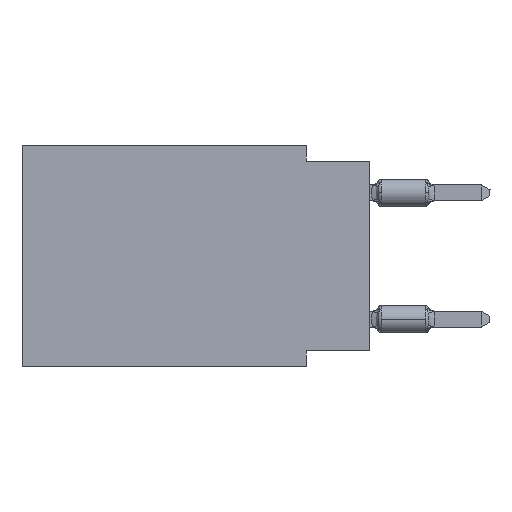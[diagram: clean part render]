
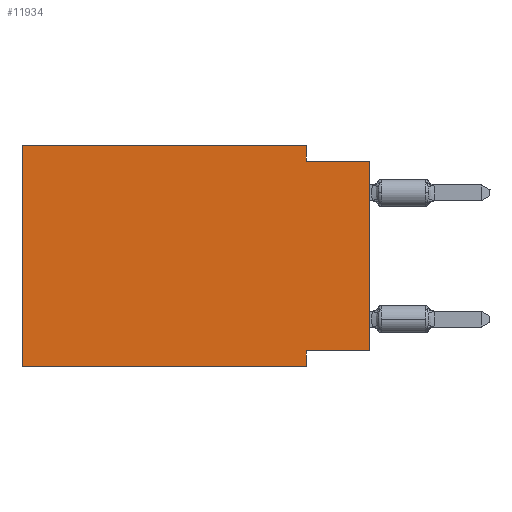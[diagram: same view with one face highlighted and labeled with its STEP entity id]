
A CAD part, left-side view. The second image highlights one B-rep face of the part: STEP entity #11934.
In plain terms, the highlighted planar face has unit normal (-1, 0, 0).
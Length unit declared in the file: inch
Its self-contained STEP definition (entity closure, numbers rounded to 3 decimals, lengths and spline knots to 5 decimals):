
#329 = CARTESIAN_POINT ( 'NONE',  ( 0., 0.55, 0. ) ) ;
#379 = DIRECTION ( 'NONE',  ( 0., -1., 0. ) ) ;
#888 = PLANE ( 'NONE',  #16378 ) ;
#1260 = DIRECTION ( 'NONE',  ( 0., 0., 1. ) ) ;
#1665 = DIRECTION ( 'NONE',  ( 0., 0., -1. ) ) ;
#2385 = EDGE_CURVE ( 'NONE', #27962, #37296, #24498, .T. ) ;
#2590 = CARTESIAN_POINT ( 'NONE',  ( 0., 0.1, 0. ) ) ;
#2630 = CARTESIAN_POINT ( 'NONE',  ( 0., 0.1, 0. ) ) ;
#3808 = CARTESIAN_POINT ( 'NONE',  ( 0., 0.1, -0.35 ) ) ;
#3850 = VERTEX_POINT ( 'NONE', #15170 ) ;
#4298 = EDGE_CURVE ( 'NONE', #32614, #6247, #18585, .T. ) ;
#4773 = EDGE_LOOP ( 'NONE', ( #17050, #33288, #7568, #12447, #37825, #22223, #14088, #26135 ) ) ;
#6037 = VERTEX_POINT ( 'NONE', #27906 ) ;
#6247 = VERTEX_POINT ( 'NONE', #2590 ) ;
#6806 = DIRECTION ( 'NONE',  ( 0., -1., 0. ) ) ;
#6886 = DIRECTION ( 'NONE',  ( 0., 0., -1. ) ) ;
#7568 = ORIENTED_EDGE ( 'NONE', *, *, #37549, .F. ) ;
#7593 = DIRECTION ( 'NONE',  ( 0., 0., 1. ) ) ;
#8701 = LINE ( 'NONE', #35371, #34907 ) ;
#9130 = VECTOR ( 'NONE', #1665, 39.37008 ) ;
#11760 = VECTOR ( 'NONE', #7593, 39.37008 ) ;
#11934 = ADVANCED_FACE ( 'NONE', ( #29723 ), #888, .F. ) ;
#12447 = ORIENTED_EDGE ( 'NONE', *, *, #4298, .F. ) ;
#12802 = LINE ( 'NONE', #31176, #11760 ) ;
#12887 = DIRECTION ( 'NONE',  ( 0., -1., 0. ) ) ;
#14088 = ORIENTED_EDGE ( 'NONE', *, *, #2385, .F. ) ;
#14455 = VECTOR ( 'NONE', #1260, 39.37008 ) ;
#14785 = DIRECTION ( 'NONE',  ( 0., 0., -1. ) ) ;
#14844 = EDGE_CURVE ( 'NONE', #34185, #6037, #36817, .T. ) ;
#15170 = CARTESIAN_POINT ( 'NONE',  ( 0., 0.55, -0.35 ) ) ;
#15378 = DIRECTION ( 'NONE',  ( 1., 0., 0. ) ) ;
#16009 = VECTOR ( 'NONE', #30143, 39.37008 ) ;
#16378 = AXIS2_PLACEMENT_3D ( 'NONE', #329, #15378, #6886 ) ;
#17050 = ORIENTED_EDGE ( 'NONE', *, *, #14844, .T. ) ;
#18198 = CARTESIAN_POINT ( 'NONE',  ( 0., 0.55, 0. ) ) ;
#18585 = LINE ( 'NONE', #19320, #33521 ) ;
#18828 = CARTESIAN_POINT ( 'NONE',  ( 0., 0., 0. ) ) ;
#18860 = CARTESIAN_POINT ( 'NONE',  ( 0., 0.1, -0.35 ) ) ;
#19320 = CARTESIAN_POINT ( 'NONE',  ( 0., 0.55, 0. ) ) ;
#19753 = VECTOR ( 'NONE', #12887, 39.37008 ) ;
#19754 = CARTESIAN_POINT ( 'NONE',  ( 0., 0., -0.325 ) ) ;
#20497 = CARTESIAN_POINT ( 'NONE',  ( 0., 0.1, -0.025 ) ) ;
#22223 = ORIENTED_EDGE ( 'NONE', *, *, #24764, .T. ) ;
#23351 = CARTESIAN_POINT ( 'NONE',  ( 0., 0.1, -0.325 ) ) ;
#24498 = LINE ( 'NONE', #18860, #9130 ) ;
#24672 = EDGE_CURVE ( 'NONE', #34185, #27962, #35767, .T. ) ;
#24764 = EDGE_CURVE ( 'NONE', #3850, #37296, #34374, .T. ) ;
#25333 = VECTOR ( 'NONE', #14785, 39.37008 ) ;
#25657 = EDGE_CURVE ( 'NONE', #3850, #32614, #12802, .T. ) ;
#26135 = ORIENTED_EDGE ( 'NONE', *, *, #24672, .F. ) ;
#26202 = LINE ( 'NONE', #2630, #25333 ) ;
#27906 = CARTESIAN_POINT ( 'NONE',  ( 0., 0., -0.025 ) ) ;
#27962 = VERTEX_POINT ( 'NONE', #23351 ) ;
#29723 = FACE_OUTER_BOUND ( 'NONE', #4773, .T. ) ;
#30143 = DIRECTION ( 'NONE',  ( 0., 1., 0. ) ) ;
#31074 = CARTESIAN_POINT ( 'NONE',  ( 0., 0.55, -0.35 ) ) ;
#31176 = CARTESIAN_POINT ( 'NONE',  ( 0., 0.55, 0. ) ) ;
#32614 = VERTEX_POINT ( 'NONE', #18198 ) ;
#32966 = EDGE_CURVE ( 'NONE', #36776, #6037, #8701, .T. ) ;
#33053 = CARTESIAN_POINT ( 'NONE',  ( 0., 0., -0.325 ) ) ;
#33288 = ORIENTED_EDGE ( 'NONE', *, *, #32966, .F. ) ;
#33521 = VECTOR ( 'NONE', #6806, 39.37008 ) ;
#34185 = VERTEX_POINT ( 'NONE', #19754 ) ;
#34374 = LINE ( 'NONE', #31074, #19753 ) ;
#34907 = VECTOR ( 'NONE', #379, 39.37008 ) ;
#35371 = CARTESIAN_POINT ( 'NONE',  ( 0., 0., -0.025 ) ) ;
#35767 = LINE ( 'NONE', #33053, #16009 ) ;
#36776 = VERTEX_POINT ( 'NONE', #20497 ) ;
#36817 = LINE ( 'NONE', #18828, #14455 ) ;
#37296 = VERTEX_POINT ( 'NONE', #3808 ) ;
#37549 = EDGE_CURVE ( 'NONE', #6247, #36776, #26202, .T. ) ;
#37825 = ORIENTED_EDGE ( 'NONE', *, *, #25657, .F. ) ;
